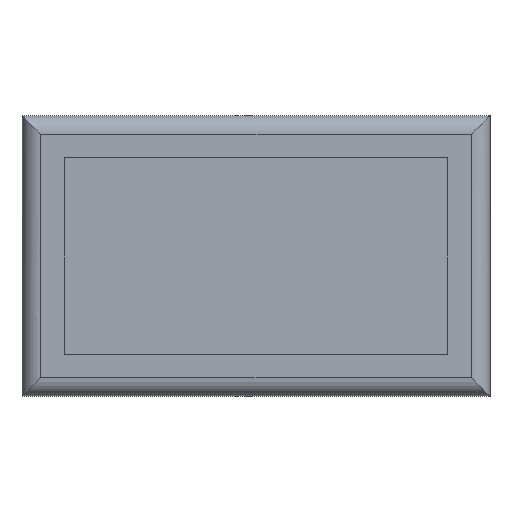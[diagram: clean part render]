
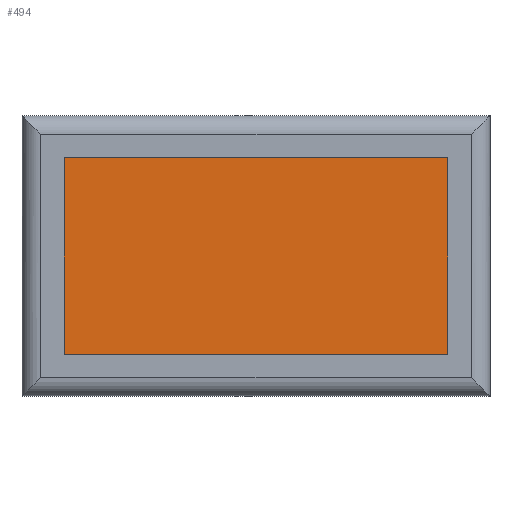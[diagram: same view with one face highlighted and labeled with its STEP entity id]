
A CAD part, left-side view. The second image highlights one B-rep face of the part: STEP entity #494.
In plain terms, the highlighted planar face has unit normal (-1, 0, 0).
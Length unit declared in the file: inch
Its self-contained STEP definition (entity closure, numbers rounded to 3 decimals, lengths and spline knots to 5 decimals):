
#1 = PLANE ( 'NONE',  #263 ) ;
#4 = VECTOR ( 'NONE', #314, 39.37008 ) ;
#10 = DIRECTION ( 'NONE',  ( -1., 0., 0. ) ) ;
#23 = DIRECTION ( 'NONE',  ( 0., -1., 0. ) ) ;
#67 = CARTESIAN_POINT ( 'NONE',  ( 0.04, 0., -1.02 ) ) ;
#69 = EDGE_CURVE ( 'NONE', #645, #577, #189, .T. ) ;
#75 = ORIENTED_EDGE ( 'NONE', *, *, #69, .T. ) ;
#103 = VECTOR ( 'NONE', #23, 39.37008 ) ;
#169 = EDGE_CURVE ( 'NONE', #616, #479, #587, .T. ) ;
#177 = FACE_OUTER_BOUND ( 'NONE', #555, .T. ) ;
#189 = LINE ( 'NONE', #626, #596 ) ;
#190 = CARTESIAN_POINT ( 'NONE',  ( 0.04, -1.82, -0.18 ) ) ;
#198 = LINE ( 'NONE', #67, #631 ) ;
#249 = DIRECTION ( 'NONE',  ( 0., -1., 0. ) ) ;
#256 = LINE ( 'NONE', #510, #103 ) ;
#263 = AXIS2_PLACEMENT_3D ( 'NONE', #569, #10, #310 ) ;
#278 = ORIENTED_EDGE ( 'NONE', *, *, #630, .F. ) ;
#310 = DIRECTION ( 'NONE',  ( 0., 0., 1. ) ) ;
#314 = DIRECTION ( 'NONE',  ( 0., 0., 1. ) ) ;
#326 = CARTESIAN_POINT ( 'NONE',  ( 0.04, -0.18, -1.02 ) ) ;
#380 = DIRECTION ( 'NONE',  ( 0., 0., 1. ) ) ;
#433 = CARTESIAN_POINT ( 'NONE',  ( 0.04, -0.18, -0.18 ) ) ;
#477 = ORIENTED_EDGE ( 'NONE', *, *, #169, .F. ) ;
#479 = VERTEX_POINT ( 'NONE', #433 ) ;
#494 = ADVANCED_FACE ( 'NONE', ( #177 ), #1, .T. ) ;
#510 = CARTESIAN_POINT ( 'NONE',  ( 0.04, 0., -0.18 ) ) ;
#514 = CARTESIAN_POINT ( 'NONE',  ( 0.04, -1.82, -1.02 ) ) ;
#538 = EDGE_CURVE ( 'NONE', #616, #645, #198, .T. ) ;
#555 = EDGE_LOOP ( 'NONE', ( #278, #477, #625, #75 ) ) ;
#569 = CARTESIAN_POINT ( 'NONE',  ( 0.04, 0., 0. ) ) ;
#577 = VERTEX_POINT ( 'NONE', #190 ) ;
#587 = LINE ( 'NONE', #760, #4 ) ;
#596 = VECTOR ( 'NONE', #380, 39.37008 ) ;
#616 = VERTEX_POINT ( 'NONE', #326 ) ;
#625 = ORIENTED_EDGE ( 'NONE', *, *, #538, .T. ) ;
#626 = CARTESIAN_POINT ( 'NONE',  ( 0.04, -1.82, 0. ) ) ;
#630 = EDGE_CURVE ( 'NONE', #479, #577, #256, .T. ) ;
#631 = VECTOR ( 'NONE', #249, 39.37008 ) ;
#645 = VERTEX_POINT ( 'NONE', #514 ) ;
#760 = CARTESIAN_POINT ( 'NONE',  ( 0.04, -0.18, 0. ) ) ;
